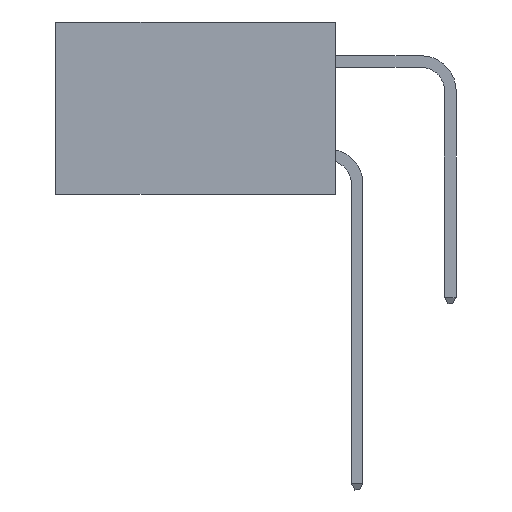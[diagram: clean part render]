
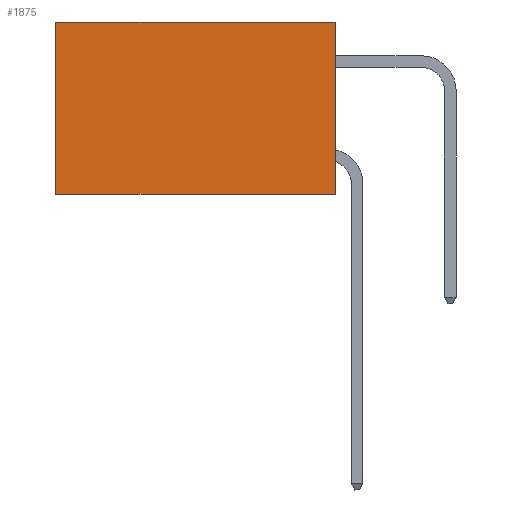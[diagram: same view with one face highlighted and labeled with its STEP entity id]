
A CAD part, left-side view. The second image highlights one B-rep face of the part: STEP entity #1875.
In plain terms, the highlighted planar face has unit normal (-1, 0, 0).
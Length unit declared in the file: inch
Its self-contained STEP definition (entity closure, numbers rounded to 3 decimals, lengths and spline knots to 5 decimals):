
#730 = ORIENTED_EDGE ( 'NONE', *, *, #2564, .T. ) ;
#764 = EDGE_CURVE ( 'NONE', #15630, #3195, #12220, .T. ) ;
#1198 = EDGE_LOOP ( 'NONE', ( #730, #8591, #6114, #4923 ) ) ;
#1875 = ADVANCED_FACE ( 'NONE', ( #18095 ), #13751, .F. ) ;
#2046 = CARTESIAN_POINT ( 'NONE',  ( 0.2875, 0.6, 0. ) ) ;
#2318 = DIRECTION ( 'NONE',  ( 0., 1., 0. ) ) ;
#2564 = EDGE_CURVE ( 'NONE', #3195, #3175, #15587, .T. ) ;
#3175 = VERTEX_POINT ( 'NONE', #5585 ) ;
#3195 = VERTEX_POINT ( 'NONE', #8471 ) ;
#3326 = AXIS2_PLACEMENT_3D ( 'NONE', #17808, #17673, #17547 ) ;
#3345 = EDGE_CURVE ( 'NONE', #15630, #17592, #17644, .T. ) ;
#3373 = CARTESIAN_POINT ( 'NONE',  ( 0.2875, 0., 0. ) ) ;
#4110 = DIRECTION ( 'NONE',  ( 0., 0., -1. ) ) ;
#4923 = ORIENTED_EDGE ( 'NONE', *, *, #764, .T. ) ;
#5585 = CARTESIAN_POINT ( 'NONE',  ( 0.2875, 0.6, -0.37 ) ) ;
#5797 = CARTESIAN_POINT ( 'NONE',  ( 0.2875, 0., -0.37 ) ) ;
#6114 = ORIENTED_EDGE ( 'NONE', *, *, #3345, .F. ) ;
#6424 = VECTOR ( 'NONE', #2318, 39.37008 ) ;
#6873 = CARTESIAN_POINT ( 'NONE',  ( 0.2875, 0., 0. ) ) ;
#7372 = DIRECTION ( 'NONE',  ( 0., 1., 0. ) ) ;
#8447 = VECTOR ( 'NONE', #7372, 39.37008 ) ;
#8471 = CARTESIAN_POINT ( 'NONE',  ( 0.2875, 0.6, 0. ) ) ;
#8591 = ORIENTED_EDGE ( 'NONE', *, *, #14431, .F. ) ;
#10807 = VECTOR ( 'NONE', #17661, 39.37008 ) ;
#11063 = VECTOR ( 'NONE', #4110, 39.37008 ) ;
#11430 = CARTESIAN_POINT ( 'NONE',  ( 0.2875, 0., 0. ) ) ;
#12220 = LINE ( 'NONE', #6873, #8447 ) ;
#12618 = CARTESIAN_POINT ( 'NONE',  ( 0.2875, 0., -0.37 ) ) ;
#13751 = PLANE ( 'NONE',  #3326 ) ;
#13980 = LINE ( 'NONE', #12618, #6424 ) ;
#14431 = EDGE_CURVE ( 'NONE', #17592, #3175, #13980, .T. ) ;
#15587 = LINE ( 'NONE', #2046, #11063 ) ;
#15630 = VERTEX_POINT ( 'NONE', #11430 ) ;
#17547 = DIRECTION ( 'NONE',  ( 0., 0., -1. ) ) ;
#17592 = VERTEX_POINT ( 'NONE', #5797 ) ;
#17644 = LINE ( 'NONE', #3373, #10807 ) ;
#17661 = DIRECTION ( 'NONE',  ( 0., 0., -1. ) ) ;
#17673 = DIRECTION ( 'NONE',  ( 1., 0., 0. ) ) ;
#17808 = CARTESIAN_POINT ( 'NONE',  ( 0.2875, 0., 0. ) ) ;
#18095 = FACE_OUTER_BOUND ( 'NONE', #1198, .T. ) ;
